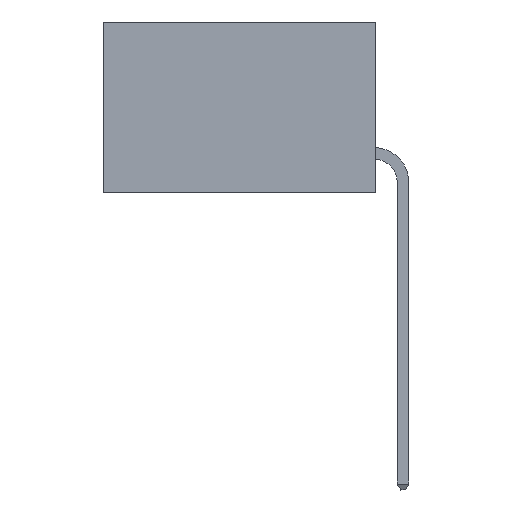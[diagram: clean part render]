
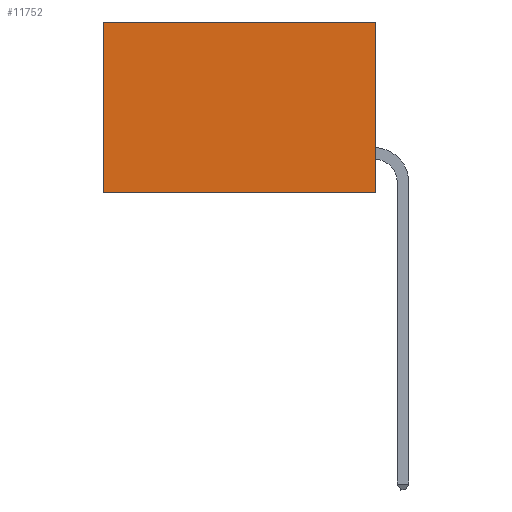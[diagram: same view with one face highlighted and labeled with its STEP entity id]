
A CAD part, left-side view. The second image highlights one B-rep face of the part: STEP entity #11752.
In plain terms, the highlighted planar face has unit normal (-1, 0, 0).
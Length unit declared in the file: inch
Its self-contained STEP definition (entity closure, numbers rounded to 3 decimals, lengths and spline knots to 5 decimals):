
#209 = ORIENTED_EDGE ( 'NONE', *, *, #14060, .T. ) ;
#232 = VERTEX_POINT ( 'NONE', #1477 ) ;
#262 = ORIENTED_EDGE ( 'NONE', *, *, #12662, .F. ) ;
#277 = ORIENTED_EDGE ( 'NONE', *, *, #10180, .F. ) ;
#332 = ORIENTED_EDGE ( 'NONE', *, *, #14510, .T. ) ;
#957 = DIRECTION ( 'NONE',  ( 0., 1., 0. ) ) ;
#1477 = CARTESIAN_POINT ( 'NONE',  ( 0.277, 0.59, -0.37 ) ) ;
#2518 = VERTEX_POINT ( 'NONE', #10744 ) ;
#3053 = DIRECTION ( 'NONE',  ( 1., 0., 0. ) ) ;
#3207 = AXIS2_PLACEMENT_3D ( 'NONE', #14117, #3053, #11718 ) ;
#3244 = LINE ( 'NONE', #13371, #12342 ) ;
#3361 = LINE ( 'NONE', #9895, #9554 ) ;
#3604 = CARTESIAN_POINT ( 'NONE',  ( 0.277, 0., 0. ) ) ;
#3811 = VERTEX_POINT ( 'NONE', #14754 ) ;
#4789 = VERTEX_POINT ( 'NONE', #10168 ) ;
#6756 = LINE ( 'NONE', #9922, #12863 ) ;
#8031 = PLANE ( 'NONE',  #3207 ) ;
#9554 = VECTOR ( 'NONE', #11134, 39.37008 ) ;
#9895 = CARTESIAN_POINT ( 'NONE',  ( 0.277, 0., -0.37 ) ) ;
#9922 = CARTESIAN_POINT ( 'NONE',  ( 0.277, 0.59, -0.37 ) ) ;
#9976 = VECTOR ( 'NONE', #957, 39.37008 ) ;
#10168 = CARTESIAN_POINT ( 'NONE',  ( 0.277, 0., -0.37 ) ) ;
#10180 = EDGE_CURVE ( 'NONE', #3811, #4789, #3361, .T. ) ;
#10744 = CARTESIAN_POINT ( 'NONE',  ( 0.277, 0.59, 0. ) ) ;
#11134 = DIRECTION ( 'NONE',  ( 0., 0., -1. ) ) ;
#11156 = DIRECTION ( 'NONE',  ( 0., 0., -1. ) ) ;
#11718 = DIRECTION ( 'NONE',  ( 0., 0., -1. ) ) ;
#11752 = ADVANCED_FACE ( 'NONE', ( #12936 ), #8031, .F. ) ;
#12342 = VECTOR ( 'NONE', #14576, 39.37008 ) ;
#12662 = EDGE_CURVE ( 'NONE', #4789, #232, #3244, .T. ) ;
#12863 = VECTOR ( 'NONE', #11156, 39.37008 ) ;
#12936 = FACE_OUTER_BOUND ( 'NONE', #13898, .T. ) ;
#13371 = CARTESIAN_POINT ( 'NONE',  ( 0.277, 0., -0.37 ) ) ;
#13898 = EDGE_LOOP ( 'NONE', ( #209, #262, #277, #332 ) ) ;
#14060 = EDGE_CURVE ( 'NONE', #2518, #232, #6756, .T. ) ;
#14117 = CARTESIAN_POINT ( 'NONE',  ( 0.277, 0., -0.37 ) ) ;
#14510 = EDGE_CURVE ( 'NONE', #3811, #2518, #16048, .T. ) ;
#14576 = DIRECTION ( 'NONE',  ( 0., 1., 0. ) ) ;
#14754 = CARTESIAN_POINT ( 'NONE',  ( 0.277, 0., 0. ) ) ;
#16048 = LINE ( 'NONE', #3604, #9976 ) ;
